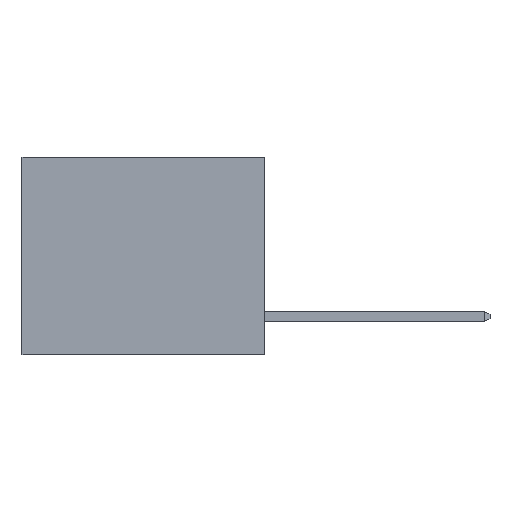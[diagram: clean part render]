
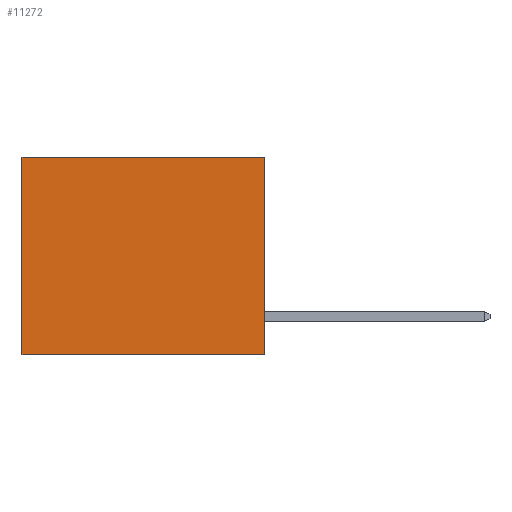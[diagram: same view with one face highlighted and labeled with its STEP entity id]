
A CAD part, left-side view. The second image highlights one B-rep face of the part: STEP entity #11272.
In plain terms, the highlighted planar face has unit normal (-1, 0, 0).
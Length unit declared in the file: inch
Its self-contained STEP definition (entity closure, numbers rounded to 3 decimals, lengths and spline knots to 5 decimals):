
#209 = DIRECTION ( 'NONE',  ( 0., 0., -1. ) ) ;
#817 = EDGE_LOOP ( 'NONE', ( #14661, #6034, #4009, #5440 ) ) ;
#974 = VECTOR ( 'NONE', #7491, 39.37008 ) ;
#1363 = FACE_OUTER_BOUND ( 'NONE', #817, .T. ) ;
#2303 = LINE ( 'NONE', #8802, #12639 ) ;
#3086 = CARTESIAN_POINT ( 'NONE',  ( 0.3165, 0.6, -0.49 ) ) ;
#3117 = CARTESIAN_POINT ( 'NONE',  ( 0.3165, 0., -0.49 ) ) ;
#3175 = VERTEX_POINT ( 'NONE', #3086 ) ;
#3404 = LINE ( 'NONE', #16635, #974 ) ;
#3836 = EDGE_CURVE ( 'NONE', #10203, #3175, #3404, .T. ) ;
#4009 = ORIENTED_EDGE ( 'NONE', *, *, #10224, .F. ) ;
#4446 = VERTEX_POINT ( 'NONE', #14756 ) ;
#4896 = VECTOR ( 'NONE', #15952, 39.37008 ) ;
#5440 = ORIENTED_EDGE ( 'NONE', *, *, #15808, .T. ) ;
#6034 = ORIENTED_EDGE ( 'NONE', *, *, #8743, .F. ) ;
#7118 = LINE ( 'NONE', #3117, #4896 ) ;
#7170 = CARTESIAN_POINT ( 'NONE',  ( 0.3165, 0., -0.49 ) ) ;
#7240 = DIRECTION ( 'NONE',  ( 1., 0., 0. ) ) ;
#7491 = DIRECTION ( 'NONE',  ( 0., 0., -1. ) ) ;
#8365 = AXIS2_PLACEMENT_3D ( 'NONE', #7170, #7240, #16212 ) ;
#8743 = EDGE_CURVE ( 'NONE', #4446, #3175, #7118, .T. ) ;
#8802 = CARTESIAN_POINT ( 'NONE',  ( 0.3165, 0., 0. ) ) ;
#8906 = VECTOR ( 'NONE', #209, 39.37008 ) ;
#9266 = VERTEX_POINT ( 'NONE', #10853 ) ;
#9337 = CARTESIAN_POINT ( 'NONE',  ( 0.3165, 0.6, 0. ) ) ;
#9916 = PLANE ( 'NONE',  #8365 ) ;
#10203 = VERTEX_POINT ( 'NONE', #9337 ) ;
#10224 = EDGE_CURVE ( 'NONE', #9266, #4446, #12732, .T. ) ;
#10643 = CARTESIAN_POINT ( 'NONE',  ( 0.3165, 0., -0.49 ) ) ;
#10853 = CARTESIAN_POINT ( 'NONE',  ( 0.3165, 0., 0. ) ) ;
#11272 = ADVANCED_FACE ( 'NONE', ( #1363 ), #9916, .F. ) ;
#12639 = VECTOR ( 'NONE', #14002, 39.37008 ) ;
#12732 = LINE ( 'NONE', #10643, #8906 ) ;
#14002 = DIRECTION ( 'NONE',  ( 0., 1., 0. ) ) ;
#14661 = ORIENTED_EDGE ( 'NONE', *, *, #3836, .T. ) ;
#14756 = CARTESIAN_POINT ( 'NONE',  ( 0.3165, 0., -0.49 ) ) ;
#15808 = EDGE_CURVE ( 'NONE', #9266, #10203, #2303, .T. ) ;
#15952 = DIRECTION ( 'NONE',  ( 0., 1., 0. ) ) ;
#16212 = DIRECTION ( 'NONE',  ( 0., 0., -1. ) ) ;
#16635 = CARTESIAN_POINT ( 'NONE',  ( 0.3165, 0.6, -0.49 ) ) ;
